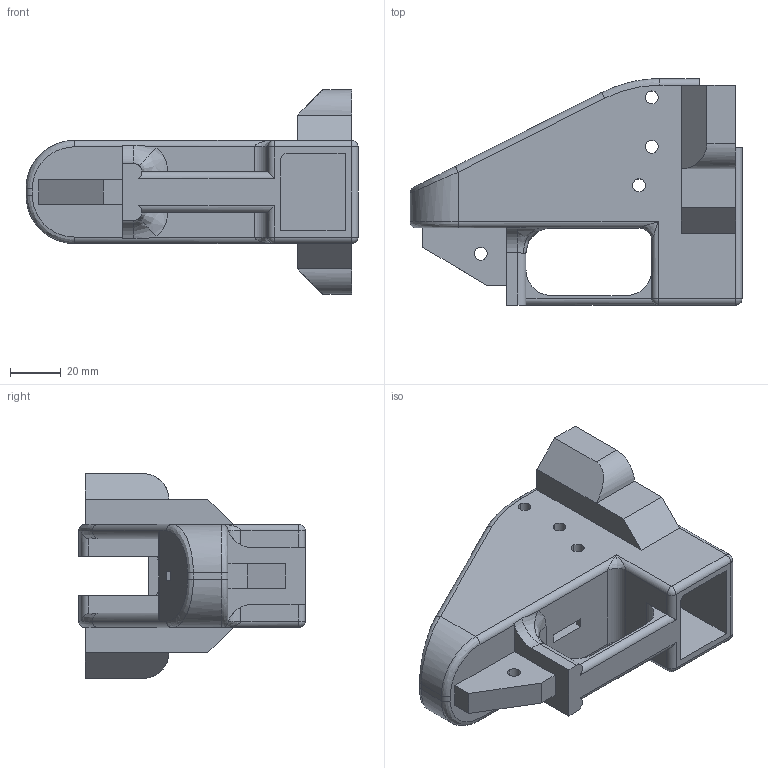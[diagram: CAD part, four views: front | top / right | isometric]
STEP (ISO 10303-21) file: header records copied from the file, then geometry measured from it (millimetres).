
FILE_DESCRIPTION (( 'STEP AP214' ), '1' );
FILE_NAME ('chamberframe.STEP', '2013-07-04T02:24:07', ( '' ), ( '' ), 'SwSTEP 2.0', 'SolidWorks 2012', '' );
FILE_SCHEMA (( 'AUTOMOTIVE_DESIGN' ));
Length unit declared in the file: millimetre
Products named in the file (1): chamberframe
Bounding box: 130.94 x 89.31 x 80.64 mm (x, y, z)
Volume: 177397.7 mm3; surface area: 51699.6 mm2
Topology: 1 solids, 1 shells, 180 faces, 487 edges, 301 vertices
Faces by surface type: plane 90, cylinder 66, bspline 16, sphere 4, cone 2, torus 2
Entity records: 6454 total; most frequent: CARTESIAN_POINT 1957, ORIENTED_EDGE 962, DIRECTION 909, EDGE_CURVE 481, AXIS2_PLACEMENT_3D 303, VECTOR 303, LINE 303, VERTEX_POINT 301
